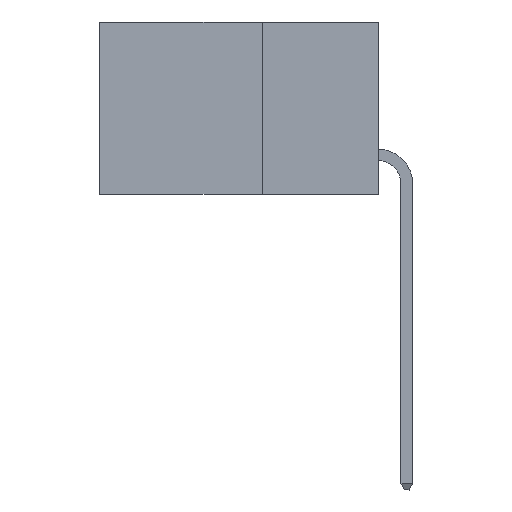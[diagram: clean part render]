
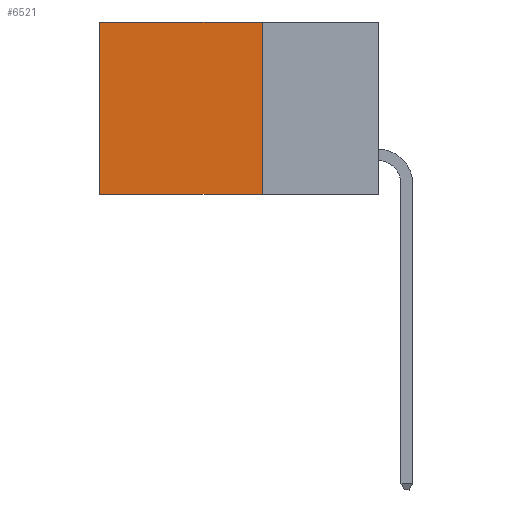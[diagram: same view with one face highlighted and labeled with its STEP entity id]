
A CAD part, left-side view. The second image highlights one B-rep face of the part: STEP entity #6521.
In plain terms, the highlighted planar face has unit normal (-1, 0, 0).
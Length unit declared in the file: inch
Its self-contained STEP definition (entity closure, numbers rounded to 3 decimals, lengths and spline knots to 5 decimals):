
#75 = EDGE_LOOP ( 'NONE', ( #6996, #9060, #8176, #4922 ) ) ;
#231 = CARTESIAN_POINT ( 'NONE',  ( 0.298, 0.6, 0. ) ) ;
#1279 = EDGE_CURVE ( 'NONE', #6970, #2970, #6657, .T. ) ;
#1640 = CARTESIAN_POINT ( 'NONE',  ( 0.298, 0.25, -0.37 ) ) ;
#1762 = EDGE_CURVE ( 'NONE', #3827, #4228, #8925, .T. ) ;
#2086 = CARTESIAN_POINT ( 'NONE',  ( 0.298, 0.25, 0. ) ) ;
#2090 = DIRECTION ( 'NONE',  ( 0., 1., 0. ) ) ;
#2970 = VERTEX_POINT ( 'NONE', #4787 ) ;
#3083 = DIRECTION ( 'NONE',  ( 1., 0., 0. ) ) ;
#3619 = FACE_OUTER_BOUND ( 'NONE', #75, .T. ) ;
#3827 = VERTEX_POINT ( 'NONE', #7934 ) ;
#4228 = VERTEX_POINT ( 'NONE', #5066 ) ;
#4673 = CARTESIAN_POINT ( 'NONE',  ( 0.298, 0.25, 0. ) ) ;
#4787 = CARTESIAN_POINT ( 'NONE',  ( 0.298, 0.6, -0.37 ) ) ;
#4922 = ORIENTED_EDGE ( 'NONE', *, *, #1762, .T. ) ;
#5037 = EDGE_CURVE ( 'NONE', #3827, #6970, #11292, .T. ) ;
#5066 = CARTESIAN_POINT ( 'NONE',  ( 0.298, 0.6, 0. ) ) ;
#5879 = CARTESIAN_POINT ( 'NONE',  ( 0.298, 0.25, -0.37 ) ) ;
#6133 = VECTOR ( 'NONE', #6880, 39.37008 ) ;
#6284 = DIRECTION ( 'NONE',  ( 0., 0., -1. ) ) ;
#6354 = VECTOR ( 'NONE', #10733, 39.37008 ) ;
#6521 = ADVANCED_FACE ( 'NONE', ( #3619 ), #7955, .F. ) ;
#6657 = LINE ( 'NONE', #1640, #11833 ) ;
#6825 = CARTESIAN_POINT ( 'NONE',  ( 0.298, 0.25, 0. ) ) ;
#6880 = DIRECTION ( 'NONE',  ( 0., 0., -1. ) ) ;
#6970 = VERTEX_POINT ( 'NONE', #5879 ) ;
#6996 = ORIENTED_EDGE ( 'NONE', *, *, #9446, .T. ) ;
#7053 = AXIS2_PLACEMENT_3D ( 'NONE', #2086, #3083, #9914 ) ;
#7934 = CARTESIAN_POINT ( 'NONE',  ( 0.298, 0.25, 0. ) ) ;
#7955 = PLANE ( 'NONE',  #7053 ) ;
#8176 = ORIENTED_EDGE ( 'NONE', *, *, #5037, .F. ) ;
#8732 = LINE ( 'NONE', #231, #11614 ) ;
#8925 = LINE ( 'NONE', #4673, #6354 ) ;
#9060 = ORIENTED_EDGE ( 'NONE', *, *, #1279, .F. ) ;
#9446 = EDGE_CURVE ( 'NONE', #4228, #2970, #8732, .T. ) ;
#9914 = DIRECTION ( 'NONE',  ( 0., 0., -1. ) ) ;
#10733 = DIRECTION ( 'NONE',  ( 0., 1., 0. ) ) ;
#11292 = LINE ( 'NONE', #6825, #6133 ) ;
#11614 = VECTOR ( 'NONE', #6284, 39.37008 ) ;
#11833 = VECTOR ( 'NONE', #2090, 39.37008 ) ;
